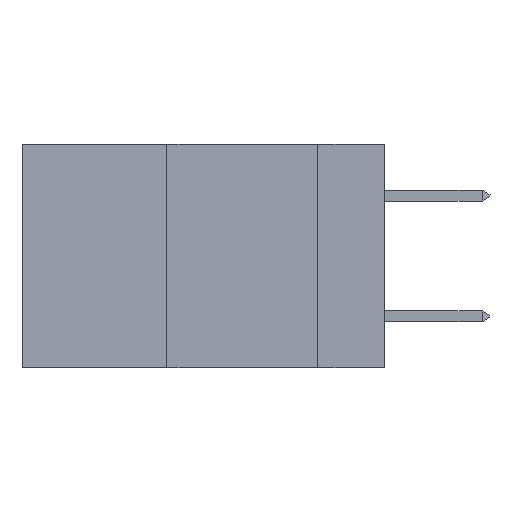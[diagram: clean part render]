
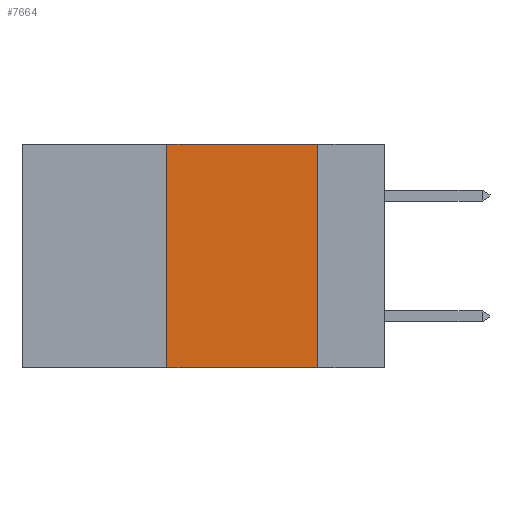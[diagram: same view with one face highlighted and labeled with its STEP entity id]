
A CAD part, left-side view. The second image highlights one B-rep face of the part: STEP entity #7664.
In plain terms, the highlighted planar face has unit normal (-1, 0, 0).
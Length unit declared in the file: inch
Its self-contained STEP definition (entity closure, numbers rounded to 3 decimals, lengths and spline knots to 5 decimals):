
#455 = LINE ( 'NONE', #8964, #2551 ) ;
#667 = EDGE_LOOP ( 'NONE', ( #4754, #6856, #4216, #6311 ) ) ;
#859 = DIRECTION ( 'NONE',  ( 0., 0., -1. ) ) ;
#943 = VERTEX_POINT ( 'NONE', #4759 ) ;
#1439 = CARTESIAN_POINT ( 'NONE',  ( 0., 0.6, -0.37 ) ) ;
#2005 = VERTEX_POINT ( 'NONE', #10972 ) ;
#2551 = VECTOR ( 'NONE', #8593, 39.37008 ) ;
#2630 = CARTESIAN_POINT ( 'NONE',  ( 0., 0.11, -0.37 ) ) ;
#3341 = VERTEX_POINT ( 'NONE', #2630 ) ;
#3781 = EDGE_CURVE ( 'NONE', #8496, #3341, #455, .T. ) ;
#4216 = ORIENTED_EDGE ( 'NONE', *, *, #5000, .F. ) ;
#4754 = ORIENTED_EDGE ( 'NONE', *, *, #3781, .F. ) ;
#4759 = CARTESIAN_POINT ( 'NONE',  ( 0., 0.36, 0. ) ) ;
#5000 = EDGE_CURVE ( 'NONE', #2005, #943, #10542, .T. ) ;
#5331 = PLANE ( 'NONE',  #9373 ) ;
#5404 = LINE ( 'NONE', #1439, #9829 ) ;
#5994 = DIRECTION ( 'NONE',  ( 0., -1., 0. ) ) ;
#6188 = VECTOR ( 'NONE', #7209, 39.37008 ) ;
#6237 = DIRECTION ( 'NONE',  ( 1., 0., 0. ) ) ;
#6311 = ORIENTED_EDGE ( 'NONE', *, *, #7888, .T. ) ;
#6771 = EDGE_CURVE ( 'NONE', #943, #8496, #10741, .T. ) ;
#6793 = CARTESIAN_POINT ( 'NONE',  ( 0., 0.6, 0. ) ) ;
#6856 = ORIENTED_EDGE ( 'NONE', *, *, #6771, .F. ) ;
#7156 = CARTESIAN_POINT ( 'NONE',  ( 0., 0.36, 0. ) ) ;
#7209 = DIRECTION ( 'NONE',  ( 0., 0., 1. ) ) ;
#7617 = DIRECTION ( 'NONE',  ( 0., -1., 0. ) ) ;
#7664 = ADVANCED_FACE ( 'NONE', ( #8361 ), #5331, .F. ) ;
#7888 = EDGE_CURVE ( 'NONE', #2005, #3341, #5404, .T. ) ;
#8361 = FACE_OUTER_BOUND ( 'NONE', #667, .T. ) ;
#8476 = CARTESIAN_POINT ( 'NONE',  ( 0., 0.11, 0. ) ) ;
#8496 = VERTEX_POINT ( 'NONE', #8476 ) ;
#8593 = DIRECTION ( 'NONE',  ( 0., 0., -1. ) ) ;
#8964 = CARTESIAN_POINT ( 'NONE',  ( 0., 0.11, 0. ) ) ;
#9373 = AXIS2_PLACEMENT_3D ( 'NONE', #11070, #6237, #859 ) ;
#9829 = VECTOR ( 'NONE', #7617, 39.37008 ) ;
#10263 = VECTOR ( 'NONE', #5994, 39.37008 ) ;
#10542 = LINE ( 'NONE', #7156, #6188 ) ;
#10741 = LINE ( 'NONE', #6793, #10263 ) ;
#10972 = CARTESIAN_POINT ( 'NONE',  ( 0., 0.36, -0.37 ) ) ;
#11070 = CARTESIAN_POINT ( 'NONE',  ( 0., 0.6, 0. ) ) ;
